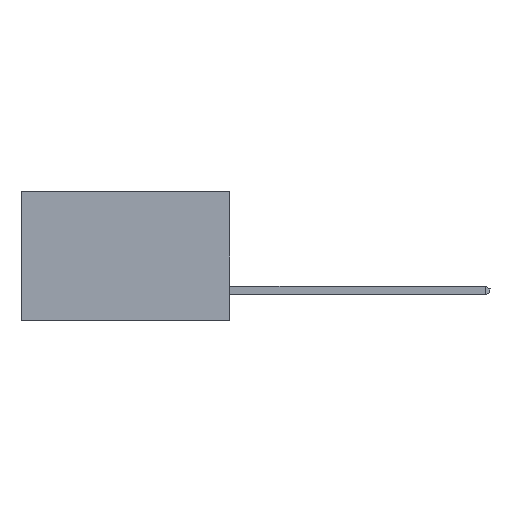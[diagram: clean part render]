
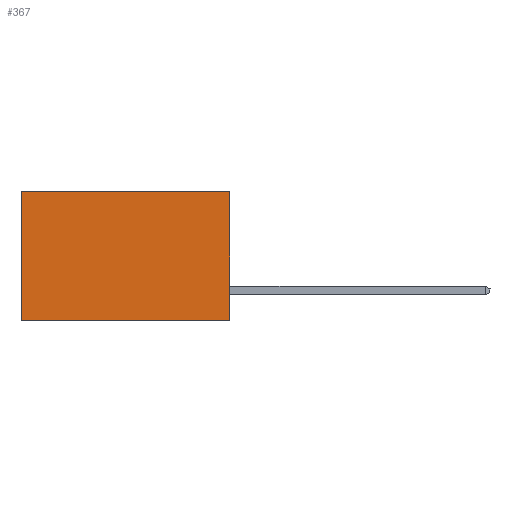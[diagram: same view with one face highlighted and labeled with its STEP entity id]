
A CAD part, left-side view. The second image highlights one B-rep face of the part: STEP entity #367.
In plain terms, the highlighted planar face has unit normal (-1, 0, 0).
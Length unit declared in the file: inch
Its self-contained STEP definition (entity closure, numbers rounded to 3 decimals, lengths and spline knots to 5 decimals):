
#367 = ADVANCED_FACE ( 'NONE', ( #11284 ), #13705, .F. ) ;
#368 = CARTESIAN_POINT ( 'NONE',  ( 0.2615, 0., 0. ) ) ;
#587 = CARTESIAN_POINT ( 'NONE',  ( 0.2615, 0., -0.37 ) ) ;
#643 = CARTESIAN_POINT ( 'NONE',  ( 0.2615, 0., -0.37 ) ) ;
#645 = DIRECTION ( 'NONE',  ( 0., 0., -1. ) ) ;
#763 = VECTOR ( 'NONE', #8653, 39.37008 ) ;
#1185 = EDGE_LOOP ( 'NONE', ( #12904, #4461, #11304, #2759 ) ) ;
#1691 = VECTOR ( 'NONE', #2323, 39.37008 ) ;
#2323 = DIRECTION ( 'NONE',  ( 0., 0., -1. ) ) ;
#2759 = ORIENTED_EDGE ( 'NONE', *, *, #7942, .T. ) ;
#3671 = VECTOR ( 'NONE', #8273, 39.37008 ) ;
#4207 = DIRECTION ( 'NONE',  ( 0., 1., 0. ) ) ;
#4421 = LINE ( 'NONE', #587, #3671 ) ;
#4461 = ORIENTED_EDGE ( 'NONE', *, *, #11994, .F. ) ;
#4725 = EDGE_CURVE ( 'NONE', #10300, #12440, #12575, .T. ) ;
#7387 = CARTESIAN_POINT ( 'NONE',  ( 0.2615, 0., -0.37 ) ) ;
#7426 = CARTESIAN_POINT ( 'NONE',  ( 0.2615, 0., -0.37 ) ) ;
#7942 = EDGE_CURVE ( 'NONE', #10300, #13976, #14238, .T. ) ;
#7985 = AXIS2_PLACEMENT_3D ( 'NONE', #7387, #15955, #645 ) ;
#8273 = DIRECTION ( 'NONE',  ( 0., 1., 0. ) ) ;
#8401 = LINE ( 'NONE', #16359, #763 ) ;
#8653 = DIRECTION ( 'NONE',  ( 0., 0., -1. ) ) ;
#9213 = CARTESIAN_POINT ( 'NONE',  ( 0.2615, 0.6, 0. ) ) ;
#9341 = VERTEX_POINT ( 'NONE', #12222 ) ;
#10300 = VERTEX_POINT ( 'NONE', #13272 ) ;
#11284 = FACE_OUTER_BOUND ( 'NONE', #1185, .T. ) ;
#11304 = ORIENTED_EDGE ( 'NONE', *, *, #4725, .F. ) ;
#11662 = VECTOR ( 'NONE', #4207, 39.37008 ) ;
#11994 = EDGE_CURVE ( 'NONE', #12440, #9341, #4421, .T. ) ;
#12222 = CARTESIAN_POINT ( 'NONE',  ( 0.2615, 0.6, -0.37 ) ) ;
#12440 = VERTEX_POINT ( 'NONE', #643 ) ;
#12575 = LINE ( 'NONE', #7426, #1691 ) ;
#12904 = ORIENTED_EDGE ( 'NONE', *, *, #13638, .T. ) ;
#13272 = CARTESIAN_POINT ( 'NONE',  ( 0.2615, 0., 0. ) ) ;
#13638 = EDGE_CURVE ( 'NONE', #13976, #9341, #8401, .T. ) ;
#13705 = PLANE ( 'NONE',  #7985 ) ;
#13976 = VERTEX_POINT ( 'NONE', #9213 ) ;
#14238 = LINE ( 'NONE', #368, #11662 ) ;
#15955 = DIRECTION ( 'NONE',  ( 1., 0., 0. ) ) ;
#16359 = CARTESIAN_POINT ( 'NONE',  ( 0.2615, 0.6, -0.37 ) ) ;
